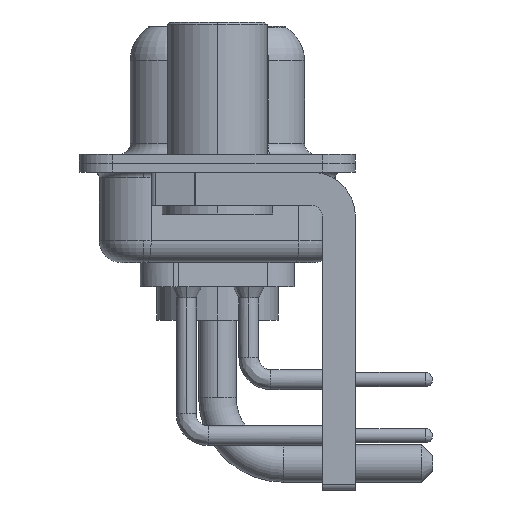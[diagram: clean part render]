
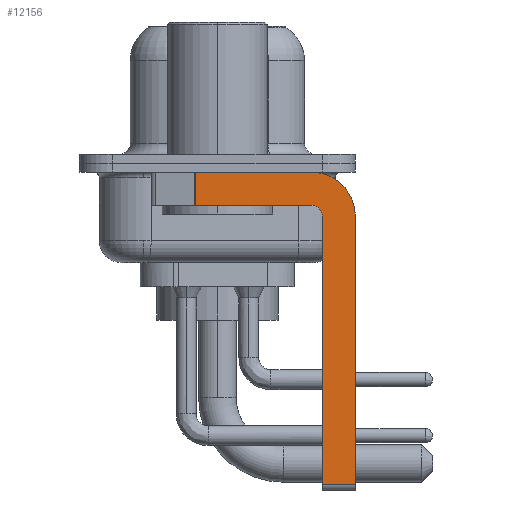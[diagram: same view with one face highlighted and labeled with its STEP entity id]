
A CAD part, left-side view. The second image highlights one B-rep face of the part: STEP entity #12156.
In plain terms, the highlighted planar face has unit normal (-1, 0, 0).
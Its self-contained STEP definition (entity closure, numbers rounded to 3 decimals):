
#25 = ORIENTED_EDGE ( 'NONE', *, *, #17777, .F. ) ;
#500 = VERTEX_POINT ( 'NONE', #6326 ) ;
#650 = DIRECTION ( 'NONE',  ( 0., 0., -1. ) ) ;
#1183 = LINE ( 'NONE', #2684, #4780 ) ;
#1216 = CIRCLE ( 'NONE', #10130, 0.5 ) ;
#1224 = FACE_OUTER_BOUND ( 'NONE', #2880, .T. ) ;
#1330 = DIRECTION ( 'NONE',  ( 1., 0., 0. ) ) ;
#1741 = CIRCLE ( 'NONE', #13754, 2. ) ;
#2032 = DIRECTION ( 'NONE',  ( 0., 0., -1. ) ) ;
#2137 = CARTESIAN_POINT ( 'NONE',  ( -2.9, -4.25, -2.4 ) ) ;
#2684 = CARTESIAN_POINT ( 'NONE',  ( -2.9, -4.75, -14.8 ) ) ;
#2880 = EDGE_LOOP ( 'NONE', ( #7621, #13676, #8664, #25, #19615, #17227, #12109, #14287 ) ) ;
#2938 = PLANE ( 'NONE',  #14513 ) ;
#3648 = DIRECTION ( 'NONE',  ( 1., 0., 0. ) ) ;
#3980 = VECTOR ( 'NONE', #16227, 1000. ) ;
#4411 = VERTEX_POINT ( 'NONE', #18781 ) ;
#4780 = VECTOR ( 'NONE', #7523, 1000. ) ;
#5098 = EDGE_CURVE ( 'NONE', #17700, #12746, #13542, .T. ) ;
#5104 = EDGE_CURVE ( 'NONE', #9861, #12746, #16762, .T. ) ;
#5384 = CARTESIAN_POINT ( 'NONE',  ( -2.9, -4.25, -14.55 ) ) ;
#5580 = CARTESIAN_POINT ( 'NONE',  ( -2.9, -6.25, -2.4 ) ) ;
#6326 = CARTESIAN_POINT ( 'NONE',  ( -2.9, 0.978, -0.4 ) ) ;
#6689 = EDGE_CURVE ( 'NONE', #17700, #14452, #1183, .T. ) ;
#6755 = CARTESIAN_POINT ( 'NONE',  ( -2.9, -4.75, -2.4 ) ) ;
#7477 = VECTOR ( 'NONE', #650, 1000. ) ;
#7523 = DIRECTION ( 'NONE',  ( 0., 0., 1. ) ) ;
#7563 = CARTESIAN_POINT ( 'NONE',  ( -2.9, -4.25, -2.4 ) ) ;
#7621 = ORIENTED_EDGE ( 'NONE', *, *, #18260, .F. ) ;
#8646 = CARTESIAN_POINT ( 'NONE',  ( -2.9, -4.75, -14.55 ) ) ;
#8664 = ORIENTED_EDGE ( 'NONE', *, *, #14258, .F. ) ;
#8977 = DIRECTION ( 'NONE',  ( -1., 0., 0. ) ) ;
#9604 = CARTESIAN_POINT ( 'NONE',  ( -2.9, 0.978, -1.9 ) ) ;
#9682 = LINE ( 'NONE', #14743, #3980 ) ;
#9730 = VECTOR ( 'NONE', #16153, 1000. ) ;
#9861 = VERTEX_POINT ( 'NONE', #5580 ) ;
#9937 = EDGE_CURVE ( 'NONE', #18644, #9861, #1741, .T. ) ;
#10080 = CARTESIAN_POINT ( 'NONE',  ( -2.9, -6.25, -14.55 ) ) ;
#10130 = AXIS2_PLACEMENT_3D ( 'NONE', #12532, #8977, #15529 ) ;
#12109 = ORIENTED_EDGE ( 'NONE', *, *, #5104, .F. ) ;
#12156 = ADVANCED_FACE ( 'NONE', ( #1224 ), #2938, .F. ) ;
#12169 = CARTESIAN_POINT ( 'NONE',  ( -2.9, -4.25, -0.4 ) ) ;
#12532 = CARTESIAN_POINT ( 'NONE',  ( -2.9, -4.25, -2.4 ) ) ;
#12746 = VERTEX_POINT ( 'NONE', #10080 ) ;
#12756 = CARTESIAN_POINT ( 'NONE',  ( -2.9, -4.25, -1.9 ) ) ;
#13542 = LINE ( 'NONE', #5384, #21147 ) ;
#13676 = ORIENTED_EDGE ( 'NONE', *, *, #16655, .T. ) ;
#13689 = CARTESIAN_POINT ( 'NONE',  ( -2.9, 3., -0.4 ) ) ;
#13754 = AXIS2_PLACEMENT_3D ( 'NONE', #2137, #3648, #2032 ) ;
#14258 = EDGE_CURVE ( 'NONE', #14690, #4411, #9682, .T. ) ;
#14287 = ORIENTED_EDGE ( 'NONE', *, *, #9937, .F. ) ;
#14452 = VERTEX_POINT ( 'NONE', #6755 ) ;
#14513 = AXIS2_PLACEMENT_3D ( 'NONE', #7563, #1330, #15726 ) ;
#14690 = VERTEX_POINT ( 'NONE', #12756 ) ;
#14743 = CARTESIAN_POINT ( 'NONE',  ( -2.9, -4.25, -1.9 ) ) ;
#15371 = DIRECTION ( 'NONE',  ( 0., -1., 0. ) ) ;
#15529 = DIRECTION ( 'NONE',  ( 0., 0., 1. ) ) ;
#15726 = DIRECTION ( 'NONE',  ( 0., 0., -1. ) ) ;
#16153 = DIRECTION ( 'NONE',  ( 0., 0., -1. ) ) ;
#16227 = DIRECTION ( 'NONE',  ( 0., 1., 0. ) ) ;
#16655 = EDGE_CURVE ( 'NONE', #500, #4411, #17762, .T. ) ;
#16762 = LINE ( 'NONE', #19862, #7477 ) ;
#17227 = ORIENTED_EDGE ( 'NONE', *, *, #5098, .T. ) ;
#17700 = VERTEX_POINT ( 'NONE', #8646 ) ;
#17762 = LINE ( 'NONE', #9604, #9730 ) ;
#17777 = EDGE_CURVE ( 'NONE', #14452, #14690, #1216, .T. ) ;
#18260 = EDGE_CURVE ( 'NONE', #500, #18644, #18827, .T. ) ;
#18644 = VERTEX_POINT ( 'NONE', #12169 ) ;
#18781 = CARTESIAN_POINT ( 'NONE',  ( -2.9, 0.978, -1.9 ) ) ;
#18827 = LINE ( 'NONE', #13689, #20748 ) ;
#19615 = ORIENTED_EDGE ( 'NONE', *, *, #6689, .F. ) ;
#19862 = CARTESIAN_POINT ( 'NONE',  ( -2.9, -6.25, -2.4 ) ) ;
#20633 = DIRECTION ( 'NONE',  ( 0., -1., 0. ) ) ;
#20748 = VECTOR ( 'NONE', #20633, 1000. ) ;
#21147 = VECTOR ( 'NONE', #15371, 1000. ) ;
